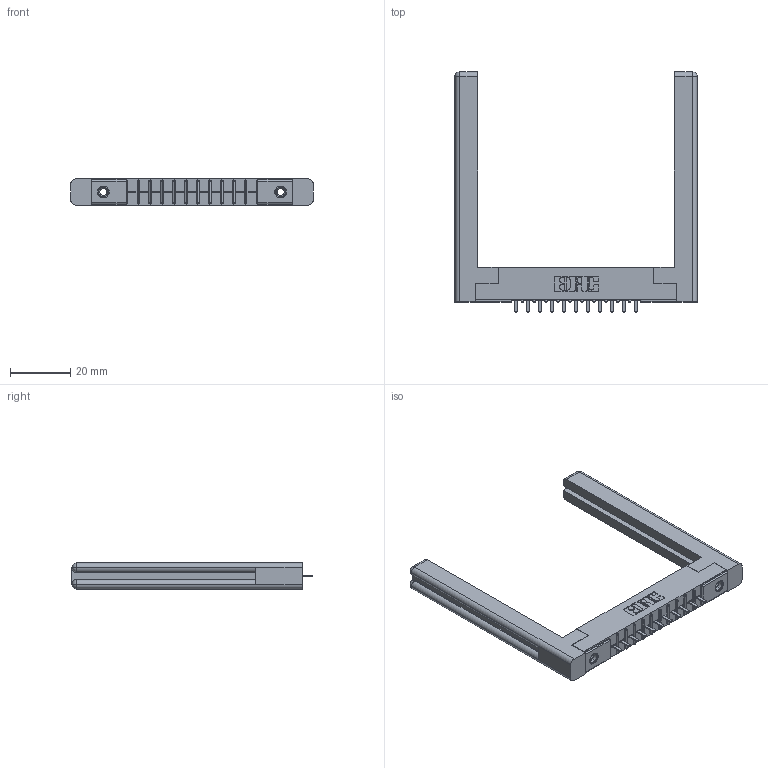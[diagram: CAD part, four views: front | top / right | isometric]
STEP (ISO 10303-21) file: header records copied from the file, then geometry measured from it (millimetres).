
FILE_DESCRIPTION (( 'STEP AP203' ), '1' );
FILE_NAME ('306-011-521-158.STEP', '2019-09-11T19:28:40', ( '' ), ( '' ), 'SwSTEP 2.0', 'SolidWorks 2016', '' );
FILE_SCHEMA (( 'CONFIG_CONTROL_DESIGN' ));
Length unit declared in the file: inch
Products named in the file (5): 306 Part_.156 Dia; 345-250-001_345-250-001-102; 306-290-001_121; 306-011-521-158; 307-220-058
Assembly tree (16 placements, depth 2):
  306-011-521-158
    306 Part_.156 Dia
    306-290-001_121  x11
    345-250-001_345-250-001-102  x2
    307-220-058  x2
Bounding box: 80.21 x 79.53 x 8.71 mm (x, y, z)
Volume: 13065.3 mm3; surface area: 12889.4 mm2
Topology: 16 solids, 16 shells, 1028 faces, 2837 edges, 1818 vertices
Faces by surface type: plane 669, cylinder 291, sphere 44, cone 12, torus 12
Entity records: 16863 total; most frequent: CARTESIAN_POINT 2835, DIRECTION 2754, ORIENTED_EDGE 2748, EDGE_CURVE 1374, VECTOR 1052, LINE 1052, VERTEX_POINT 878, AXIS2_PLACEMENT_3D 851
